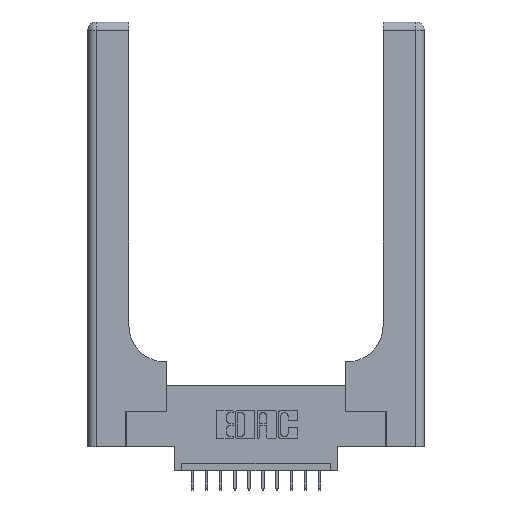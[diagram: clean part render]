
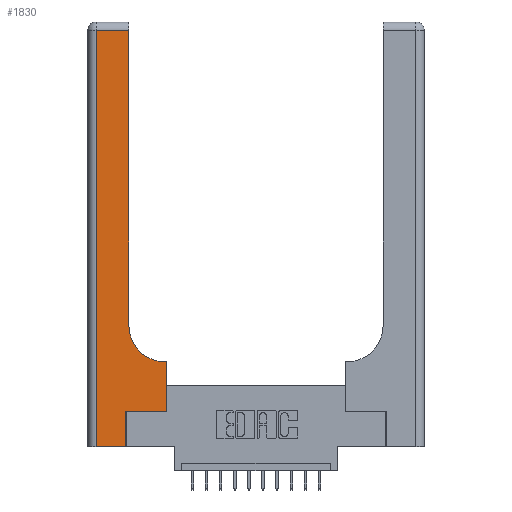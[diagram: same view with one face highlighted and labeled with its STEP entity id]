
A CAD part, top view. The second image highlights one B-rep face of the part: STEP entity #1830.
In plain terms, the highlighted planar face has unit normal (0, 0, 1).
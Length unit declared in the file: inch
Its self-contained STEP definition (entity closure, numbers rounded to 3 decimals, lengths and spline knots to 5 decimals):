
#38 = EDGE_CURVE ( 'NONE', #17011, #13623, #3182, .T. ) ;
#127 = CARTESIAN_POINT ( 'NONE',  ( 0.06, 2.94, 0.37 ) ) ;
#198 = DIRECTION ( 'NONE',  ( 1., 0., 0. ) ) ;
#214 = ORIENTED_EDGE ( 'NONE', *, *, #16964, .T. ) ;
#352 = LINE ( 'NONE', #12278, #12353 ) ;
#398 = CARTESIAN_POINT ( 'NONE',  ( 0.269, 0., 0.37 ) ) ;
#826 = VERTEX_POINT ( 'NONE', #4424 ) ;
#1054 = DIRECTION ( 'NONE',  ( 0., 0., -1. ) ) ;
#1137 = DIRECTION ( 'NONE',  ( 0., 0., -1. ) ) ;
#1227 = DIRECTION ( 'NONE',  ( -1., 0., 0. ) ) ;
#1369 = LINE ( 'NONE', #6752, #10633 ) ;
#1398 = DIRECTION ( 'NONE',  ( -1., 0., 0. ) ) ;
#1436 = VERTEX_POINT ( 'NONE', #127 ) ;
#1775 = AXIS2_PLACEMENT_3D ( 'NONE', #3837, #1054, #1398 ) ;
#1830 = ADVANCED_FACE ( 'NONE', ( #10628 ), #3756, .F. ) ;
#3148 = CARTESIAN_POINT ( 'NONE',  ( 0.269, 0.25, 0.37 ) ) ;
#3182 = CIRCLE ( 'NONE', #4822, 0.25 ) ;
#3577 = VECTOR ( 'NONE', #13609, 39.37008 ) ;
#3756 = PLANE ( 'NONE',  #1775 ) ;
#3765 = EDGE_LOOP ( 'NONE', ( #13796, #16753, #9550, #214, #7247, #5170, #12240, #4407, #13892 ) ) ;
#3837 = CARTESIAN_POINT ( 'NONE',  ( 0., 3., 0.37 ) ) ;
#4350 = LINE ( 'NONE', #7055, #3577 ) ;
#4407 = ORIENTED_EDGE ( 'NONE', *, *, #10672, .T. ) ;
#4424 = CARTESIAN_POINT ( 'NONE',  ( 0.06, 0., 0.37 ) ) ;
#4558 = VERTEX_POINT ( 'NONE', #5114 ) ;
#4807 = VECTOR ( 'NONE', #1227, 39.37008 ) ;
#4822 = AXIS2_PLACEMENT_3D ( 'NONE', #13086, #1137, #198 ) ;
#5114 = CARTESIAN_POINT ( 'NONE',  ( 0.5585, 0.25, 0.37 ) ) ;
#5170 = ORIENTED_EDGE ( 'NONE', *, *, #7547, .T. ) ;
#5585 = VECTOR ( 'NONE', #10828, 39.37008 ) ;
#5774 = EDGE_CURVE ( 'NONE', #1436, #826, #4350, .T. ) ;
#5860 = CARTESIAN_POINT ( 'NONE',  ( 0.269, 0.25, 0.37 ) ) ;
#6752 = CARTESIAN_POINT ( 'NONE',  ( 0.269, 0., 0.37 ) ) ;
#6796 = CARTESIAN_POINT ( 'NONE',  ( 0.2915, 3., 0.37 ) ) ;
#6808 = EDGE_CURVE ( 'NONE', #8747, #1436, #8414, .T. ) ;
#6883 = VERTEX_POINT ( 'NONE', #8756 ) ;
#7055 = CARTESIAN_POINT ( 'NONE',  ( 0.06, 3., 0.37 ) ) ;
#7247 = ORIENTED_EDGE ( 'NONE', *, *, #9524, .T. ) ;
#7547 = EDGE_CURVE ( 'NONE', #14076, #4558, #8378, .T. ) ;
#7571 = CARTESIAN_POINT ( 'NONE',  ( 0.2915, 0.85, 0.37 ) ) ;
#8177 = DIRECTION ( 'NONE',  ( 0., 1., 0. ) ) ;
#8281 = DIRECTION ( 'NONE',  ( 0., 1., 0. ) ) ;
#8378 = LINE ( 'NONE', #3148, #5585 ) ;
#8414 = LINE ( 'NONE', #14887, #15860 ) ;
#8465 = CARTESIAN_POINT ( 'NONE',  ( 0.2915, 2.94, 0.37 ) ) ;
#8480 = LINE ( 'NONE', #13814, #12175 ) ;
#8747 = VERTEX_POINT ( 'NONE', #8465 ) ;
#8756 = CARTESIAN_POINT ( 'NONE',  ( 0.5585, 0.6, 0.37 ) ) ;
#8776 = EDGE_CURVE ( 'NONE', #13623, #8747, #11009, .T. ) ;
#9524 = EDGE_CURVE ( 'NONE', #13120, #14076, #1369, .T. ) ;
#9550 = ORIENTED_EDGE ( 'NONE', *, *, #5774, .T. ) ;
#10381 = LINE ( 'NONE', #15880, #4807 ) ;
#10628 = FACE_OUTER_BOUND ( 'NONE', #3765, .T. ) ;
#10633 = VECTOR ( 'NONE', #8177, 39.37008 ) ;
#10672 = EDGE_CURVE ( 'NONE', #6883, #17011, #10381, .T. ) ;
#10828 = DIRECTION ( 'NONE',  ( 1., 0., 0. ) ) ;
#11009 = LINE ( 'NONE', #6796, #12303 ) ;
#11044 = EDGE_CURVE ( 'NONE', #4558, #6883, #352, .T. ) ;
#11184 = DIRECTION ( 'NONE',  ( 0., 1., 0. ) ) ;
#12175 = VECTOR ( 'NONE', #12494, 39.37008 ) ;
#12240 = ORIENTED_EDGE ( 'NONE', *, *, #11044, .T. ) ;
#12278 = CARTESIAN_POINT ( 'NONE',  ( 0.5585, 0.25, 0.37 ) ) ;
#12303 = VECTOR ( 'NONE', #11184, 39.37008 ) ;
#12353 = VECTOR ( 'NONE', #8281, 39.37008 ) ;
#12432 = DIRECTION ( 'NONE',  ( -1., 0., 0. ) ) ;
#12494 = DIRECTION ( 'NONE',  ( 1., 0., 0. ) ) ;
#13086 = CARTESIAN_POINT ( 'NONE',  ( 0.5415, 0.85, 0.37 ) ) ;
#13120 = VERTEX_POINT ( 'NONE', #398 ) ;
#13609 = DIRECTION ( 'NONE',  ( 0., -1., 0. ) ) ;
#13623 = VERTEX_POINT ( 'NONE', #7571 ) ;
#13796 = ORIENTED_EDGE ( 'NONE', *, *, #8776, .T. ) ;
#13814 = CARTESIAN_POINT ( 'NONE',  ( 0., 0., 0.37 ) ) ;
#13892 = ORIENTED_EDGE ( 'NONE', *, *, #38, .T. ) ;
#14076 = VERTEX_POINT ( 'NONE', #5860 ) ;
#14887 = CARTESIAN_POINT ( 'NONE',  ( 0., 2.94, 0.37 ) ) ;
#15860 = VECTOR ( 'NONE', #12432, 39.37008 ) ;
#15880 = CARTESIAN_POINT ( 'NONE',  ( 0.2915, 0.6, 0.37 ) ) ;
#16683 = CARTESIAN_POINT ( 'NONE',  ( 0.5415, 0.6, 0.37 ) ) ;
#16753 = ORIENTED_EDGE ( 'NONE', *, *, #6808, .T. ) ;
#16964 = EDGE_CURVE ( 'NONE', #826, #13120, #8480, .T. ) ;
#17011 = VERTEX_POINT ( 'NONE', #16683 ) ;
